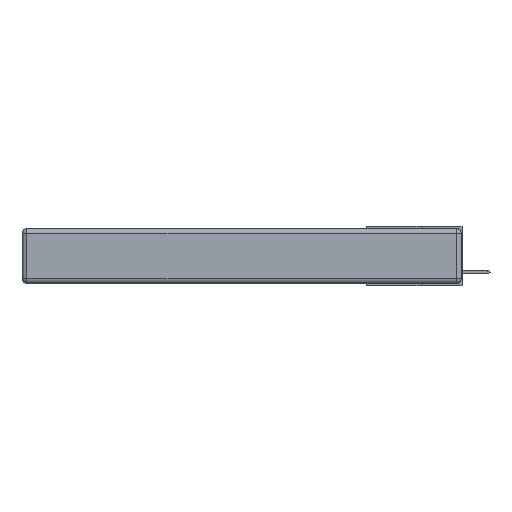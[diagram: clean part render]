
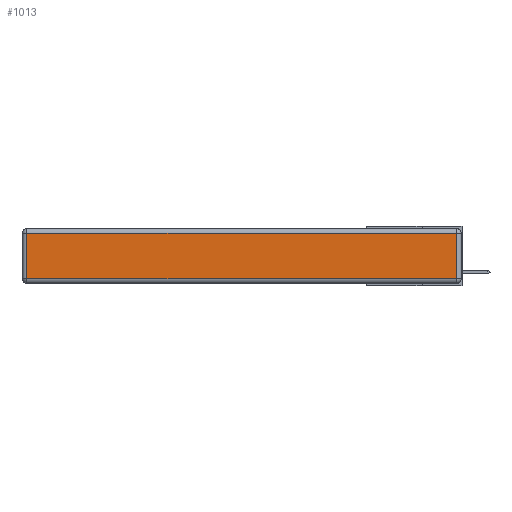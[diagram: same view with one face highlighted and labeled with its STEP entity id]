
A CAD part, left-side view. The second image highlights one B-rep face of the part: STEP entity #1013.
In plain terms, the highlighted planar face has unit normal (-1, 0, 0).
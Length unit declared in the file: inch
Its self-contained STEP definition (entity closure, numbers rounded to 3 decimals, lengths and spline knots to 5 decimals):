
#1013 = ADVANCED_FACE ( 'NONE', ( #11594 ), #11812, .T. ) ;
#1662 = EDGE_CURVE ( 'NONE', #12343, #4357, #13636, .T. ) ;
#1716 = ORIENTED_EDGE ( 'NONE', *, *, #3369, .T. ) ;
#1947 = AXIS2_PLACEMENT_3D ( 'NONE', #12912, #11648, #6965 ) ;
#2922 = VECTOR ( 'NONE', #7421, 39.37008 ) ;
#3198 = ORIENTED_EDGE ( 'NONE', *, *, #6224, .T. ) ;
#3369 = EDGE_CURVE ( 'NONE', #4340, #9427, #10627, .T. ) ;
#3414 = VECTOR ( 'NONE', #7165, 39.37008 ) ;
#3502 = ORIENTED_EDGE ( 'NONE', *, *, #1662, .T. ) ;
#4317 = VECTOR ( 'NONE', #11311, 39.37008 ) ;
#4340 = VERTEX_POINT ( 'NONE', #12430 ) ;
#4357 = VERTEX_POINT ( 'NONE', #6522 ) ;
#4385 = CARTESIAN_POINT ( 'NONE',  ( 0., 0.03, -0.03 ) ) ;
#4489 = LINE ( 'NONE', #6437, #4317 ) ;
#4821 = CARTESIAN_POINT ( 'NONE',  ( 0., 2.75, -0.03 ) ) ;
#5533 = VECTOR ( 'NONE', #7529, 39.37008 ) ;
#6224 = EDGE_CURVE ( 'NONE', #4357, #4340, #4489, .T. ) ;
#6437 = CARTESIAN_POINT ( 'NONE',  ( 0., 2.72, -0.343 ) ) ;
#6522 = CARTESIAN_POINT ( 'NONE',  ( 0., 2.72, -0.03 ) ) ;
#6965 = DIRECTION ( 'NONE',  ( 0., 0., 1. ) ) ;
#7165 = DIRECTION ( 'NONE',  ( 0., 0., 1. ) ) ;
#7421 = DIRECTION ( 'NONE',  ( 0., -1., 0. ) ) ;
#7529 = DIRECTION ( 'NONE',  ( 0., 1., 0. ) ) ;
#9427 = VERTEX_POINT ( 'NONE', #13851 ) ;
#10627 = LINE ( 'NONE', #14620, #2922 ) ;
#11153 = EDGE_LOOP ( 'NONE', ( #1716, #15061, #3502, #3198 ) ) ;
#11311 = DIRECTION ( 'NONE',  ( 0., 0., -1. ) ) ;
#11594 = FACE_OUTER_BOUND ( 'NONE', #11153, .T. ) ;
#11648 = DIRECTION ( 'NONE',  ( -1., 0., 0. ) ) ;
#11812 = PLANE ( 'NONE',  #1947 ) ;
#11999 = EDGE_CURVE ( 'NONE', #9427, #12343, #14931, .T. ) ;
#12343 = VERTEX_POINT ( 'NONE', #4385 ) ;
#12430 = CARTESIAN_POINT ( 'NONE',  ( 0., 2.72, -0.313 ) ) ;
#12912 = CARTESIAN_POINT ( 'NONE',  ( 0., 0., -0.343 ) ) ;
#13636 = LINE ( 'NONE', #4821, #5533 ) ;
#13851 = CARTESIAN_POINT ( 'NONE',  ( 0., 0.03, -0.313 ) ) ;
#14408 = CARTESIAN_POINT ( 'NONE',  ( 0., 0.03, -0.343 ) ) ;
#14620 = CARTESIAN_POINT ( 'NONE',  ( 0., 0., -0.313 ) ) ;
#14931 = LINE ( 'NONE', #14408, #3414 ) ;
#15061 = ORIENTED_EDGE ( 'NONE', *, *, #11999, .T. ) ;
